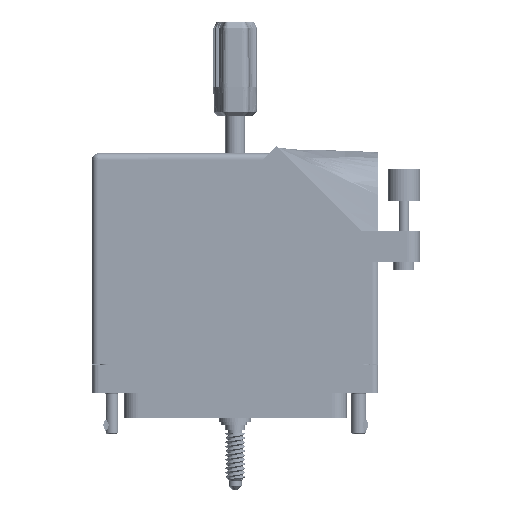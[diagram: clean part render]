
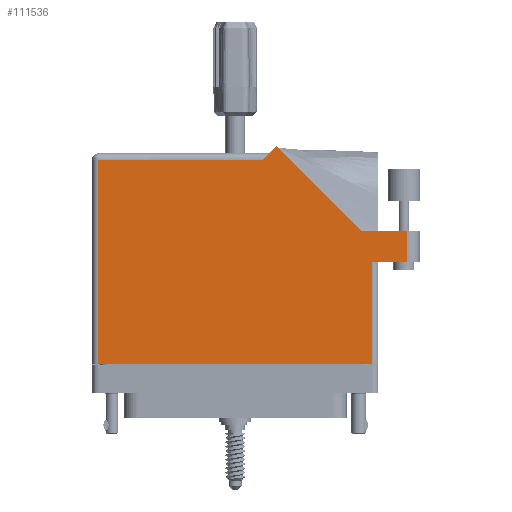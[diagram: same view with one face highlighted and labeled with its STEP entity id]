
A CAD part, front view. The second image highlights one B-rep face of the part: STEP entity #111536.
In plain terms, the highlighted face is planar.
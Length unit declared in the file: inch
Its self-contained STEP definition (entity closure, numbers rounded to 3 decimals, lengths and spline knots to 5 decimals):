
#1319 = EDGE_CURVE ( 'NONE', #49224, #84301, #77438, .T. ) ;
#2841 = VERTEX_POINT ( 'NONE', #37325 ) ;
#3744 = LINE ( 'NONE', #11095, #90481 ) ;
#6673 = CARTESIAN_POINT ( 'NONE',  ( -1.3775, -0.1, 0.765 ) ) ;
#9321 = CARTESIAN_POINT ( 'NONE',  ( 1.6525, 0.88, 0.765 ) ) ;
#10327 = EDGE_CURVE ( 'NONE', #90673, #49224, #18453, .T. ) ;
#11095 = CARTESIAN_POINT ( 'NONE',  ( 1.7775, 1.187, 0.765 ) ) ;
#13514 = LINE ( 'NONE', #55746, #73479 ) ;
#14639 = ORIENTED_EDGE ( 'NONE', *, *, #52117, .T. ) ;
#16021 = CARTESIAN_POINT ( 'NONE',  ( 0.2655, 1.868, 0.765 ) ) ;
#16142 = AXIS2_PLACEMENT_3D ( 'NONE', #35413, #72033, #62674 ) ;
#16230 = CARTESIAN_POINT ( 'NONE',  ( 1.3155, 0.88, 0.765 ) ) ;
#17023 = DIRECTION ( 'NONE',  ( -0.707, 0.707, 0. ) ) ;
#17765 = PLANE ( 'NONE',  #16142 ) ;
#18453 = LINE ( 'NONE', #6673, #109450 ) ;
#23193 = ORIENTED_EDGE ( 'NONE', *, *, #70728, .T. ) ;
#25684 = CARTESIAN_POINT ( 'NONE',  ( 1.21192, 1.187, 0.765 ) ) ;
#26132 = LINE ( 'NONE', #37804, #108633 ) ;
#27353 = VECTOR ( 'NONE', #88105, 39.37008 ) ;
#28011 = EDGE_CURVE ( 'NONE', #42374, #32900, #26132, .T. ) ;
#32900 = VERTEX_POINT ( 'NONE', #66881 ) ;
#34437 = ORIENTED_EDGE ( 'NONE', *, *, #1319, .T. ) ;
#35413 = CARTESIAN_POINT ( 'NONE',  ( -1.3775, 1.93, 0.765 ) ) ;
#35476 = EDGE_LOOP ( 'NONE', ( #77557, #100133, #53578, #14639, #23193, #83590, #102590, #77687, #34437 ) ) ;
#37325 = CARTESIAN_POINT ( 'NONE',  ( 1.21192, 1.187, 0.765 ) ) ;
#37804 = CARTESIAN_POINT ( 'NONE',  ( -1.3775, 1.868, 0.765 ) ) ;
#40439 = VERTEX_POINT ( 'NONE', #73396 ) ;
#41265 = CARTESIAN_POINT ( 'NONE',  ( 1.3155, 0.88, 0.765 ) ) ;
#42374 = VERTEX_POINT ( 'NONE', #16021 ) ;
#47558 = FACE_OUTER_BOUND ( 'NONE', #35476, .T. ) ;
#47745 = VERTEX_POINT ( 'NONE', #9321 ) ;
#49224 = VERTEX_POINT ( 'NONE', #65620 ) ;
#52117 = EDGE_CURVE ( 'NONE', #2841, #40439, #84969, .T. ) ;
#52410 = EDGE_CURVE ( 'NONE', #54224, #2841, #3744, .T. ) ;
#52721 = VECTOR ( 'NONE', #64751, 39.37008 ) ;
#53578 = ORIENTED_EDGE ( 'NONE', *, *, #52410, .T. ) ;
#53641 = VECTOR ( 'NONE', #112037, 39.37008 ) ;
#54197 = VECTOR ( 'NONE', #17023, 39.37008 ) ;
#54224 = VERTEX_POINT ( 'NONE', #90414 ) ;
#55746 = CARTESIAN_POINT ( 'NONE',  ( -1.3155, -0.1, 0.765 ) ) ;
#61350 = DIRECTION ( 'NONE',  ( 1., 0., 0. ) ) ;
#62674 = DIRECTION ( 'NONE',  ( -1., 0., 0. ) ) ;
#63098 = DIRECTION ( 'NONE',  ( 1., 0., 0. ) ) ;
#63524 = LINE ( 'NONE', #99496, #101262 ) ;
#63969 = EDGE_CURVE ( 'NONE', #84301, #47745, #63524, .T. ) ;
#64751 = DIRECTION ( 'NONE',  ( -0.707, -0.707, 0. ) ) ;
#65620 = CARTESIAN_POINT ( 'NONE',  ( 1.3155, -0.1, 0.765 ) ) ;
#66881 = CARTESIAN_POINT ( 'NONE',  ( -1.3155, 1.868, 0.765 ) ) ;
#70728 = EDGE_CURVE ( 'NONE', #40439, #42374, #114258, .T. ) ;
#72033 = DIRECTION ( 'NONE',  ( 0., 0., -1. ) ) ;
#72553 = DIRECTION ( 'NONE',  ( -1., 0., 0. ) ) ;
#73396 = CARTESIAN_POINT ( 'NONE',  ( 0.39821, 2.00071, 0.765 ) ) ;
#73469 = LINE ( 'NONE', #96756, #27353 ) ;
#73479 = VECTOR ( 'NONE', #110522, 39.37008 ) ;
#77438 = LINE ( 'NONE', #41265, #53641 ) ;
#77557 = ORIENTED_EDGE ( 'NONE', *, *, #63969, .T. ) ;
#77687 = ORIENTED_EDGE ( 'NONE', *, *, #10327, .T. ) ;
#83590 = ORIENTED_EDGE ( 'NONE', *, *, #28011, .T. ) ;
#84301 = VERTEX_POINT ( 'NONE', #16230 ) ;
#84969 = LINE ( 'NONE', #25684, #54197 ) ;
#88105 = DIRECTION ( 'NONE',  ( 0., 1., 0. ) ) ;
#89588 = EDGE_CURVE ( 'NONE', #32900, #90673, #13514, .T. ) ;
#90414 = CARTESIAN_POINT ( 'NONE',  ( 1.6525, 1.187, 0.765 ) ) ;
#90481 = VECTOR ( 'NONE', #99828, 39.37008 ) ;
#90673 = VERTEX_POINT ( 'NONE', #93316 ) ;
#93316 = CARTESIAN_POINT ( 'NONE',  ( -1.3155, -0.1, 0.765 ) ) ;
#96756 = CARTESIAN_POINT ( 'NONE',  ( 1.6525, 1.187, 0.765 ) ) ;
#99496 = CARTESIAN_POINT ( 'NONE',  ( 1.3775, 0.88, 0.765 ) ) ;
#99828 = DIRECTION ( 'NONE',  ( -1., 0., 0. ) ) ;
#100133 = ORIENTED_EDGE ( 'NONE', *, *, #103134, .T. ) ;
#101262 = VECTOR ( 'NONE', #63098, 39.37008 ) ;
#102590 = ORIENTED_EDGE ( 'NONE', *, *, #89588, .T. ) ;
#103134 = EDGE_CURVE ( 'NONE', #47745, #54224, #73469, .T. ) ;
#108617 = CARTESIAN_POINT ( 'NONE',  ( 0.3275, 1.93, 0.765 ) ) ;
#108633 = VECTOR ( 'NONE', #72553, 39.37008 ) ;
#109450 = VECTOR ( 'NONE', #61350, 39.37008 ) ;
#110522 = DIRECTION ( 'NONE',  ( 0., -1., 0. ) ) ;
#111536 = ADVANCED_FACE ( 'NONE', ( #47558 ), #17765, .F. ) ;
#112037 = DIRECTION ( 'NONE',  ( 0., 1., 0. ) ) ;
#114258 = LINE ( 'NONE', #108617, #52721 ) ;
